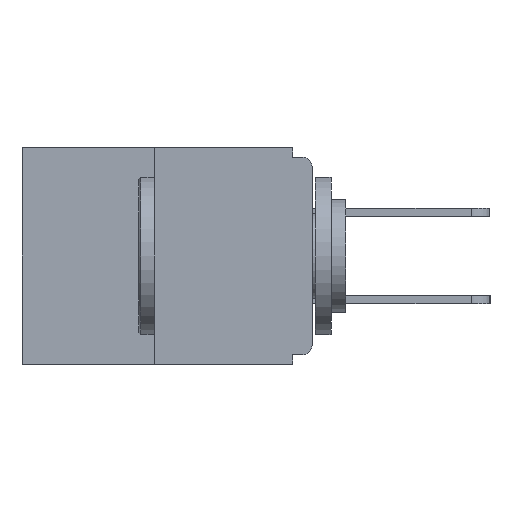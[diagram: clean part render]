
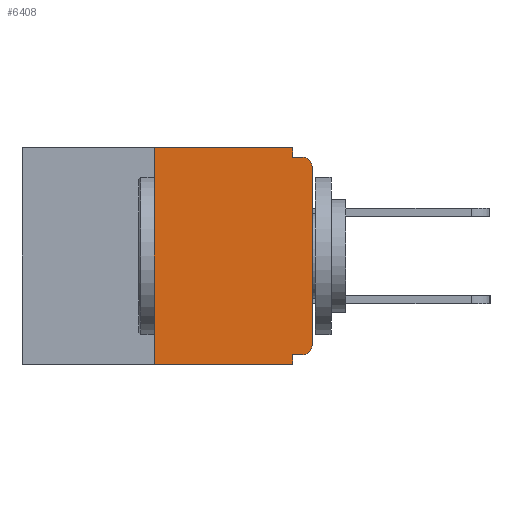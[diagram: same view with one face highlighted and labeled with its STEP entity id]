
A CAD part, left-side view. The second image highlights one B-rep face of the part: STEP entity #6408.
In plain terms, the highlighted planar face has unit normal (-1, 0, 0).
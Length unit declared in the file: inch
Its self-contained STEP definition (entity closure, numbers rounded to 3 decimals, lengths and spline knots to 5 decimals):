
#238 = FACE_OUTER_BOUND ( 'NONE', #13221, .T. ) ;
#963 = VERTEX_POINT ( 'NONE', #13855 ) ;
#1052 = DIRECTION ( 'NONE',  ( 0., 0., -1. ) ) ;
#1157 = LINE ( 'NONE', #4603, #9417 ) ;
#1172 = LINE ( 'NONE', #2825, #13011 ) ;
#1226 = ORIENTED_EDGE ( 'NONE', *, *, #1984, .F. ) ;
#1230 = AXIS2_PLACEMENT_3D ( 'NONE', #6947, #1570, #10461 ) ;
#1333 = EDGE_CURVE ( 'NONE', #3854, #963, #7941, .T. ) ;
#1393 = AXIS2_PLACEMENT_3D ( 'NONE', #7939, #12332, #10161 ) ;
#1463 = ORIENTED_EDGE ( 'NONE', *, *, #3680, .F. ) ;
#1570 = DIRECTION ( 'NONE',  ( 1., 0., 0. ) ) ;
#1984 = EDGE_CURVE ( 'NONE', #10016, #963, #8662, .T. ) ;
#2041 = CARTESIAN_POINT ( 'NONE',  ( 0., 0.25, 0. ) ) ;
#2284 = CARTESIAN_POINT ( 'NONE',  ( 0., 0.46, 0. ) ) ;
#2409 = PLANE ( 'NONE',  #1230 ) ;
#2520 = LINE ( 'NONE', #8874, #5944 ) ;
#2535 = DIRECTION ( 'NONE',  ( 0., -1., 0. ) ) ;
#2546 = LINE ( 'NONE', #10830, #10803 ) ;
#2697 = VECTOR ( 'NONE', #13770, 39.37008 ) ;
#2773 = VECTOR ( 'NONE', #4636, 39.37008 ) ;
#2825 = CARTESIAN_POINT ( 'NONE',  ( 0., 0., 0. ) ) ;
#2913 = EDGE_CURVE ( 'NONE', #7975, #12268, #2520, .T. ) ;
#3269 = CARTESIAN_POINT ( 'NONE',  ( 0., 0.015, -0.03 ) ) ;
#3680 = EDGE_CURVE ( 'NONE', #4906, #10016, #2546, .T. ) ;
#3854 = VERTEX_POINT ( 'NONE', #13154 ) ;
#4250 = DIRECTION ( 'NONE',  ( 0., 0., -1. ) ) ;
#4327 = LINE ( 'NONE', #2284, #2697 ) ;
#4603 = CARTESIAN_POINT ( 'NONE',  ( 0., 0.46, -0.343 ) ) ;
#4636 = DIRECTION ( 'NONE',  ( 0., 0., 1. ) ) ;
#4781 = LINE ( 'NONE', #10106, #10872 ) ;
#4849 = AXIS2_PLACEMENT_3D ( 'NONE', #3269, #9010, #4250 ) ;
#4906 = VERTEX_POINT ( 'NONE', #8330 ) ;
#5250 = ORIENTED_EDGE ( 'NONE', *, *, #2913, .F. ) ;
#5483 = CARTESIAN_POINT ( 'NONE',  ( 0., 0.015, -0.328 ) ) ;
#5944 = VECTOR ( 'NONE', #12265, 39.37008 ) ;
#5959 = CARTESIAN_POINT ( 'NONE',  ( 0., 0., -0.015 ) ) ;
#6253 = DIRECTION ( 'NONE',  ( 0., 0., -1. ) ) ;
#6370 = ORIENTED_EDGE ( 'NONE', *, *, #14784, .T. ) ;
#6408 = ADVANCED_FACE ( 'NONE', ( #238 ), #2409, .F. ) ;
#6947 = CARTESIAN_POINT ( 'NONE',  ( 0., 0.46, 0. ) ) ;
#7005 = CARTESIAN_POINT ( 'NONE',  ( 0., 0.031, -0.015 ) ) ;
#7169 = ORIENTED_EDGE ( 'NONE', *, *, #13627, .T. ) ;
#7463 = CIRCLE ( 'NONE', #1393, 0.015 ) ;
#7691 = ORIENTED_EDGE ( 'NONE', *, *, #8790, .F. ) ;
#7851 = ORIENTED_EDGE ( 'NONE', *, *, #13792, .F. ) ;
#7939 = CARTESIAN_POINT ( 'NONE',  ( 0., 0.015, -0.313 ) ) ;
#7941 = CIRCLE ( 'NONE', #4849, 0.015 ) ;
#7975 = VERTEX_POINT ( 'NONE', #5483 ) ;
#8090 = VERTEX_POINT ( 'NONE', #2041 ) ;
#8330 = CARTESIAN_POINT ( 'NONE',  ( 0., 0.031, 0. ) ) ;
#8662 = LINE ( 'NONE', #5959, #9379 ) ;
#8790 = EDGE_CURVE ( 'NONE', #8090, #4906, #4327, .T. ) ;
#8874 = CARTESIAN_POINT ( 'NONE',  ( 0., 0., -0.328 ) ) ;
#8886 = ORIENTED_EDGE ( 'NONE', *, *, #12505, .T. ) ;
#9010 = DIRECTION ( 'NONE',  ( -1., 0., 0. ) ) ;
#9379 = VECTOR ( 'NONE', #2535, 39.37008 ) ;
#9417 = VECTOR ( 'NONE', #13602, 39.37008 ) ;
#9726 = ORIENTED_EDGE ( 'NONE', *, *, #13601, .F. ) ;
#10016 = VERTEX_POINT ( 'NONE', #7005 ) ;
#10106 = CARTESIAN_POINT ( 'NONE',  ( 0., 0.031, -0.343 ) ) ;
#10161 = DIRECTION ( 'NONE',  ( 0., 0., -1. ) ) ;
#10461 = DIRECTION ( 'NONE',  ( 0., 0., -1. ) ) ;
#10672 = CARTESIAN_POINT ( 'NONE',  ( 0., 0.25, -0.343 ) ) ;
#10753 = VERTEX_POINT ( 'NONE', #10672 ) ;
#10803 = VECTOR ( 'NONE', #6253, 39.37008 ) ;
#10830 = CARTESIAN_POINT ( 'NONE',  ( 0., 0.031, 0. ) ) ;
#10872 = VECTOR ( 'NONE', #1052, 39.37008 ) ;
#11755 = ORIENTED_EDGE ( 'NONE', *, *, #1333, .T. ) ;
#12265 = DIRECTION ( 'NONE',  ( 0., 1., 0. ) ) ;
#12268 = VERTEX_POINT ( 'NONE', #13955 ) ;
#12332 = DIRECTION ( 'NONE',  ( -1., 0., 0. ) ) ;
#12505 = EDGE_CURVE ( 'NONE', #13400, #3854, #1172, .T. ) ;
#13011 = VECTOR ( 'NONE', #13099, 39.37008 ) ;
#13099 = DIRECTION ( 'NONE',  ( 0., 0., 1. ) ) ;
#13154 = CARTESIAN_POINT ( 'NONE',  ( 0., 0., -0.03 ) ) ;
#13178 = LINE ( 'NONE', #13678, #2773 ) ;
#13221 = EDGE_LOOP ( 'NONE', ( #7691, #7851, #6370, #9726, #5250, #7169, #8886, #11755, #1226, #1463 ) ) ;
#13396 = VERTEX_POINT ( 'NONE', #14684 ) ;
#13400 = VERTEX_POINT ( 'NONE', #14582 ) ;
#13601 = EDGE_CURVE ( 'NONE', #12268, #13396, #4781, .T. ) ;
#13602 = DIRECTION ( 'NONE',  ( 0., -1., 0. ) ) ;
#13627 = EDGE_CURVE ( 'NONE', #7975, #13400, #7463, .T. ) ;
#13678 = CARTESIAN_POINT ( 'NONE',  ( 0., 0.25, 0. ) ) ;
#13770 = DIRECTION ( 'NONE',  ( 0., -1., 0. ) ) ;
#13792 = EDGE_CURVE ( 'NONE', #10753, #8090, #13178, .T. ) ;
#13855 = CARTESIAN_POINT ( 'NONE',  ( 0., 0.015, -0.015 ) ) ;
#13955 = CARTESIAN_POINT ( 'NONE',  ( 0., 0.031, -0.328 ) ) ;
#14582 = CARTESIAN_POINT ( 'NONE',  ( 0., 0., -0.313 ) ) ;
#14684 = CARTESIAN_POINT ( 'NONE',  ( 0., 0.031, -0.343 ) ) ;
#14784 = EDGE_CURVE ( 'NONE', #10753, #13396, #1157, .T. ) ;
